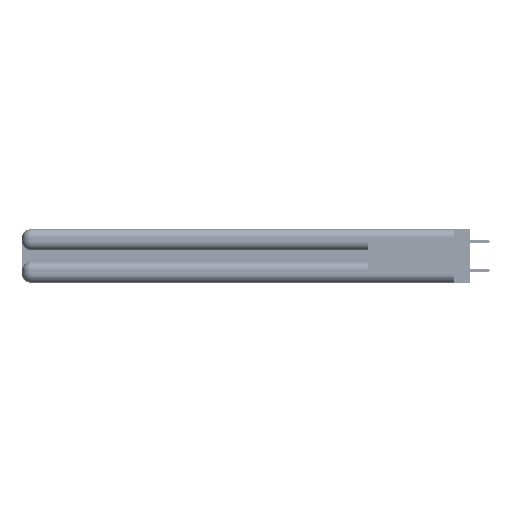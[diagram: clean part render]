
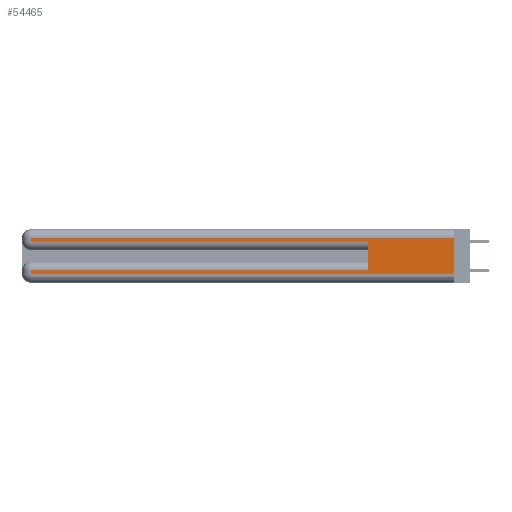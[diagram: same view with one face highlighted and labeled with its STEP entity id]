
A CAD part, left-side view. The second image highlights one B-rep face of the part: STEP entity #54465.
In plain terms, the highlighted planar face has unit normal (-1, 0, 0).
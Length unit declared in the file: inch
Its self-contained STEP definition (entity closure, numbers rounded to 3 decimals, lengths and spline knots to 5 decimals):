
#96 = VERTEX_POINT ( 'NONE', #45858 ) ;
#456 = EDGE_CURVE ( 'NONE', #25319, #96, #4396, .T. ) ;
#2664 = CARTESIAN_POINT ( 'NONE',  ( 0., 2.94, 0.06 ) ) ;
#4396 = LINE ( 'NONE', #4950, #6465 ) ;
#4950 = CARTESIAN_POINT ( 'NONE',  ( 0., 0.6, 0.145 ) ) ;
#5889 = ORIENTED_EDGE ( 'NONE', *, *, #456, .F. ) ;
#5930 = VECTOR ( 'NONE', #38569, 39.37008 ) ;
#6343 = LINE ( 'NONE', #37330, #40485 ) ;
#6465 = VECTOR ( 'NONE', #31031, 39.37008 ) ;
#7369 = CARTESIAN_POINT ( 'NONE',  ( 0., 0., 0.06 ) ) ;
#8251 = CARTESIAN_POINT ( 'NONE',  ( 0., 0.6, 0.085 ) ) ;
#8735 = CARTESIAN_POINT ( 'NONE',  ( 0., 0., 0.37 ) ) ;
#9666 = CARTESIAN_POINT ( 'NONE',  ( 0., 2.94, 0.31 ) ) ;
#11603 = VERTEX_POINT ( 'NONE', #37694 ) ;
#12756 = CARTESIAN_POINT ( 'NONE',  ( 0., 2.94, 0.37 ) ) ;
#13254 = CARTESIAN_POINT ( 'NONE',  ( 0., 0., 0.085 ) ) ;
#19670 = VECTOR ( 'NONE', #33894, 39.37008 ) ;
#21185 = CARTESIAN_POINT ( 'NONE',  ( 0., 0., 0.285 ) ) ;
#22916 = VECTOR ( 'NONE', #29497, 39.37008 ) ;
#24010 = DIRECTION ( 'NONE',  ( 0., 0., -1. ) ) ;
#25319 = VERTEX_POINT ( 'NONE', #8251 ) ;
#25726 = LINE ( 'NONE', #51776, #22916 ) ;
#26420 = DIRECTION ( 'NONE',  ( 0., 0., -1. ) ) ;
#26767 = ORIENTED_EDGE ( 'NONE', *, *, #27859, .T. ) ;
#27313 = EDGE_CURVE ( 'NONE', #33599, #45517, #38073, .T. ) ;
#27859 = EDGE_CURVE ( 'NONE', #11603, #96, #44037, .T. ) ;
#29081 = EDGE_LOOP ( 'NONE', ( #32433, #33288, #35064, #26767, #5889, #32198, #46442, #29191 ) ) ;
#29191 = ORIENTED_EDGE ( 'NONE', *, *, #27313, .T. ) ;
#29341 = VERTEX_POINT ( 'NONE', #54154 ) ;
#29497 = DIRECTION ( 'NONE',  ( 0., 0., -1. ) ) ;
#30923 = EDGE_CURVE ( 'NONE', #29341, #50643, #55331, .T. ) ;
#31031 = DIRECTION ( 'NONE',  ( 0., 0., 1. ) ) ;
#32198 = ORIENTED_EDGE ( 'NONE', *, *, #36080, .T. ) ;
#32343 = CARTESIAN_POINT ( 'NONE',  ( 0., 2.94, 0.085 ) ) ;
#32433 = ORIENTED_EDGE ( 'NONE', *, *, #48196, .F. ) ;
#33288 = ORIENTED_EDGE ( 'NONE', *, *, #30923, .T. ) ;
#33599 = VERTEX_POINT ( 'NONE', #2664 ) ;
#33894 = DIRECTION ( 'NONE',  ( 0., 1., 0. ) ) ;
#34503 = LINE ( 'NONE', #12756, #52995 ) ;
#34738 = VECTOR ( 'NONE', #43674, 39.37008 ) ;
#35064 = ORIENTED_EDGE ( 'NONE', *, *, #56174, .T. ) ;
#35559 = LINE ( 'NONE', #13254, #34738 ) ;
#36080 = EDGE_CURVE ( 'NONE', #25319, #36213, #35559, .T. ) ;
#36213 = VERTEX_POINT ( 'NONE', #32343 ) ;
#37330 = CARTESIAN_POINT ( 'NONE',  ( 0., 2.94, 0.37 ) ) ;
#37694 = CARTESIAN_POINT ( 'NONE',  ( 0., 2.94, 0.285 ) ) ;
#38073 = LINE ( 'NONE', #7369, #46650 ) ;
#38569 = DIRECTION ( 'NONE',  ( 0., -1., 0. ) ) ;
#40324 = EDGE_CURVE ( 'NONE', #36213, #33599, #6343, .T. ) ;
#40485 = VECTOR ( 'NONE', #24010, 39.37008 ) ;
#42433 = DIRECTION ( 'NONE',  ( 0., -1., 0. ) ) ;
#42854 = CARTESIAN_POINT ( 'NONE',  ( 0., 0., 0.31 ) ) ;
#43674 = DIRECTION ( 'NONE',  ( 0., 1., 0. ) ) ;
#43840 = CARTESIAN_POINT ( 'NONE',  ( 0., 0., 0.06 ) ) ;
#44037 = LINE ( 'NONE', #21185, #5930 ) ;
#45517 = VERTEX_POINT ( 'NONE', #43840 ) ;
#45858 = CARTESIAN_POINT ( 'NONE',  ( 0., 0.6, 0.285 ) ) ;
#46442 = ORIENTED_EDGE ( 'NONE', *, *, #40324, .T. ) ;
#46650 = VECTOR ( 'NONE', #42433, 39.37008 ) ;
#47866 = PLANE ( 'NONE',  #56573 ) ;
#48083 = DIRECTION ( 'NONE',  ( 0., 0., -1. ) ) ;
#48196 = EDGE_CURVE ( 'NONE', #29341, #45517, #25726, .T. ) ;
#50643 = VERTEX_POINT ( 'NONE', #9666 ) ;
#51776 = CARTESIAN_POINT ( 'NONE',  ( 0., 0., 0.37 ) ) ;
#52995 = VECTOR ( 'NONE', #48083, 39.37008 ) ;
#54154 = CARTESIAN_POINT ( 'NONE',  ( 0., 0., 0.31 ) ) ;
#54465 = ADVANCED_FACE ( 'NONE', ( #56551 ), #47866, .F. ) ;
#55331 = LINE ( 'NONE', #42854, #19670 ) ;
#56174 = EDGE_CURVE ( 'NONE', #50643, #11603, #34503, .T. ) ;
#56551 = FACE_OUTER_BOUND ( 'NONE', #29081, .T. ) ;
#56573 = AXIS2_PLACEMENT_3D ( 'NONE', #8735, #57134, #26420 ) ;
#57134 = DIRECTION ( 'NONE',  ( 1., 0., 0. ) ) ;
